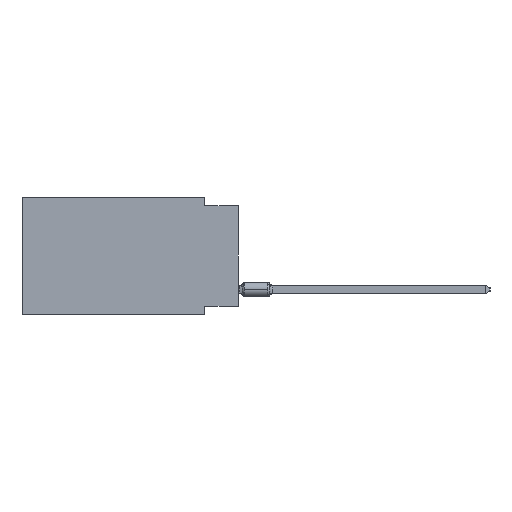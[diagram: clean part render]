
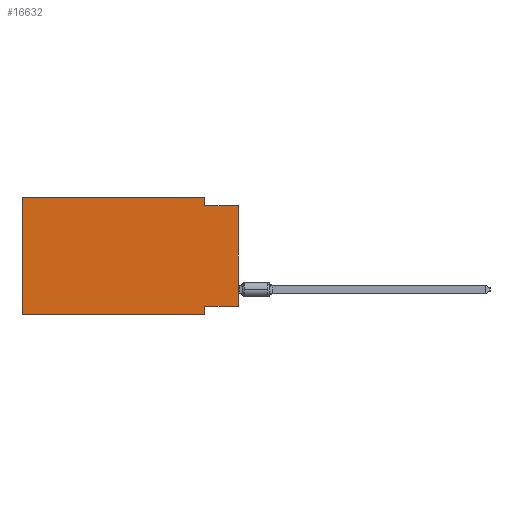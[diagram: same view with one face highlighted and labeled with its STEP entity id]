
A CAD part, left-side view. The second image highlights one B-rep face of the part: STEP entity #16632.
In plain terms, the highlighted planar face has unit normal (-1, 0, 0).
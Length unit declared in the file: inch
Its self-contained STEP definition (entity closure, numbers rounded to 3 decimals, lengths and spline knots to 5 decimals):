
#657 = CARTESIAN_POINT ( 'NONE',  ( 0., 0.1, 0. ) ) ;
#827 = CARTESIAN_POINT ( 'NONE',  ( 0., 0.1, -0.325 ) ) ;
#1095 = CARTESIAN_POINT ( 'NONE',  ( 0., 0., -0.325 ) ) ;
#1727 = PLANE ( 'NONE',  #26228 ) ;
#1842 = CARTESIAN_POINT ( 'NONE',  ( 0., 0.1, -0.35 ) ) ;
#2970 = ORIENTED_EDGE ( 'NONE', *, *, #15947, .F. ) ;
#3129 = EDGE_CURVE ( 'NONE', #28492, #17130, #7010, .T. ) ;
#3867 = CARTESIAN_POINT ( 'NONE',  ( 0., 0.645, 0. ) ) ;
#4003 = VERTEX_POINT ( 'NONE', #28716 ) ;
#5357 = DIRECTION ( 'NONE',  ( 0., -1., 0. ) ) ;
#5654 = CARTESIAN_POINT ( 'NONE',  ( 0., 0., -0.325 ) ) ;
#6964 = CARTESIAN_POINT ( 'NONE',  ( 0., 0.645, 0. ) ) ;
#7010 = LINE ( 'NONE', #37961, #19238 ) ;
#7883 = DIRECTION ( 'NONE',  ( 0., 0., -1. ) ) ;
#7946 = DIRECTION ( 'NONE',  ( 0., 0., -1. ) ) ;
#8481 = EDGE_CURVE ( 'NONE', #27577, #31802, #22202, .T. ) ;
#9513 = LINE ( 'NONE', #3867, #25023 ) ;
#9668 = ORIENTED_EDGE ( 'NONE', *, *, #13796, .T. ) ;
#10086 = DIRECTION ( 'NONE',  ( 0., -1., 0. ) ) ;
#13201 = CARTESIAN_POINT ( 'NONE',  ( 0., 0.645, 0. ) ) ;
#13436 = DIRECTION ( 'NONE',  ( 0., -1., 0. ) ) ;
#13796 = EDGE_CURVE ( 'NONE', #26357, #4003, #38349, .T. ) ;
#14179 = LINE ( 'NONE', #1095, #16164 ) ;
#14587 = EDGE_CURVE ( 'NONE', #21406, #4003, #32225, .T. ) ;
#14813 = EDGE_CURVE ( 'NONE', #32477, #21406, #14179, .T. ) ;
#15947 = EDGE_CURVE ( 'NONE', #31802, #28492, #35311, .T. ) ;
#16164 = VECTOR ( 'NONE', #34900, 39.37008 ) ;
#16278 = LINE ( 'NONE', #16678, #29993 ) ;
#16344 = DIRECTION ( 'NONE',  ( 0., 0., 1. ) ) ;
#16632 = ADVANCED_FACE ( 'NONE', ( #29294 ), #1727, .F. ) ;
#16678 = CARTESIAN_POINT ( 'NONE',  ( 0., 0., 0. ) ) ;
#17070 = VECTOR ( 'NONE', #10086, 39.37008 ) ;
#17130 = VERTEX_POINT ( 'NONE', #36217 ) ;
#19238 = VECTOR ( 'NONE', #13436, 39.37008 ) ;
#19507 = ORIENTED_EDGE ( 'NONE', *, *, #14587, .F. ) ;
#20479 = CARTESIAN_POINT ( 'NONE',  ( 0., 0.645, -0.35 ) ) ;
#21406 = VERTEX_POINT ( 'NONE', #827 ) ;
#22202 = LINE ( 'NONE', #22808, #17070 ) ;
#22808 = CARTESIAN_POINT ( 'NONE',  ( 0., 0.645, 0. ) ) ;
#25023 = VECTOR ( 'NONE', #16344, 39.37008 ) ;
#25497 = DIRECTION ( 'NONE',  ( 1., 0., 0. ) ) ;
#26228 = AXIS2_PLACEMENT_3D ( 'NONE', #13201, #25497, #28895 ) ;
#26299 = ORIENTED_EDGE ( 'NONE', *, *, #30710, .F. ) ;
#26357 = VERTEX_POINT ( 'NONE', #26599 ) ;
#26458 = VECTOR ( 'NONE', #7883, 39.37008 ) ;
#26599 = CARTESIAN_POINT ( 'NONE',  ( 0., 0.645, -0.35 ) ) ;
#27123 = ORIENTED_EDGE ( 'NONE', *, *, #8481, .F. ) ;
#27577 = VERTEX_POINT ( 'NONE', #6964 ) ;
#28074 = VECTOR ( 'NONE', #7946, 39.37008 ) ;
#28492 = VERTEX_POINT ( 'NONE', #34338 ) ;
#28716 = CARTESIAN_POINT ( 'NONE',  ( 0., 0.1, -0.35 ) ) ;
#28895 = DIRECTION ( 'NONE',  ( 0., 0., -1. ) ) ;
#29294 = FACE_OUTER_BOUND ( 'NONE', #32947, .T. ) ;
#29993 = VECTOR ( 'NONE', #38189, 39.37008 ) ;
#30710 = EDGE_CURVE ( 'NONE', #26357, #27577, #9513, .T. ) ;
#31802 = VERTEX_POINT ( 'NONE', #657 ) ;
#32225 = LINE ( 'NONE', #1842, #26458 ) ;
#32477 = VERTEX_POINT ( 'NONE', #5654 ) ;
#32492 = CARTESIAN_POINT ( 'NONE',  ( 0., 0.1, 0. ) ) ;
#32947 = EDGE_LOOP ( 'NONE', ( #39665, #36374, #2970, #27123, #26299, #9668, #19507, #39759 ) ) ;
#34338 = CARTESIAN_POINT ( 'NONE',  ( 0., 0.1, -0.025 ) ) ;
#34900 = DIRECTION ( 'NONE',  ( 0., 1., 0. ) ) ;
#35311 = LINE ( 'NONE', #32492, #28074 ) ;
#36217 = CARTESIAN_POINT ( 'NONE',  ( 0., 0., -0.025 ) ) ;
#36374 = ORIENTED_EDGE ( 'NONE', *, *, #3129, .F. ) ;
#37459 = EDGE_CURVE ( 'NONE', #32477, #17130, #16278, .T. ) ;
#37961 = CARTESIAN_POINT ( 'NONE',  ( 0., 0., -0.025 ) ) ;
#38189 = DIRECTION ( 'NONE',  ( 0., 0., 1. ) ) ;
#38349 = LINE ( 'NONE', #20479, #38667 ) ;
#38667 = VECTOR ( 'NONE', #5357, 39.37008 ) ;
#39665 = ORIENTED_EDGE ( 'NONE', *, *, #37459, .T. ) ;
#39759 = ORIENTED_EDGE ( 'NONE', *, *, #14813, .F. ) ;
